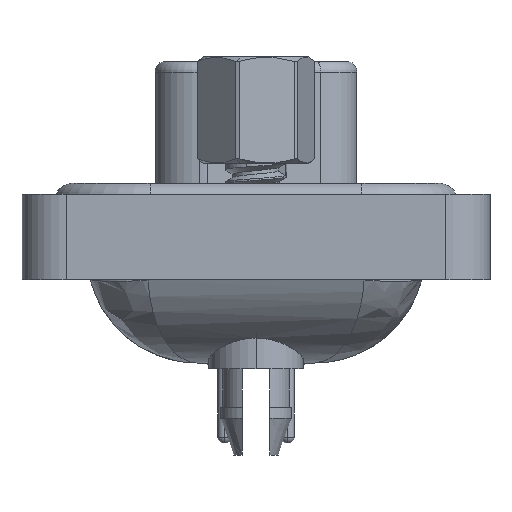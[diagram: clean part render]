
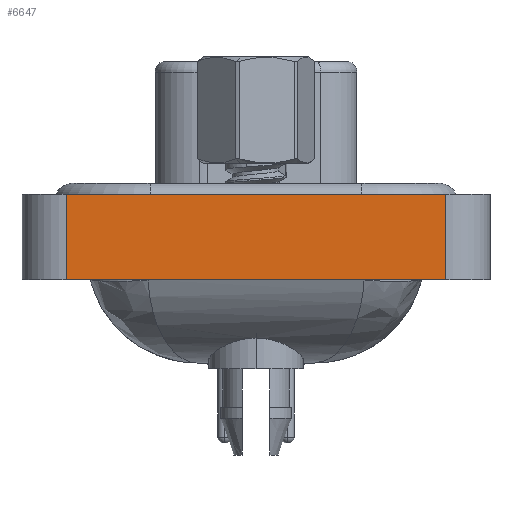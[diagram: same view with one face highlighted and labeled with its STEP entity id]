
A CAD part, left-side view. The second image highlights one B-rep face of the part: STEP entity #6647.
In plain terms, the highlighted planar face has unit normal (-1, 0, 0).
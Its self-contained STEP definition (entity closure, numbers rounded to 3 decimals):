
#2953 = EDGE_LOOP ( 'NONE', ( #7243, #8491, #27881, #7110 ) ) ;
#3103 = VERTEX_POINT ( 'NONE', #6133 ) ;
#4012 = FACE_OUTER_BOUND ( 'NONE', #2953, .T. ) ;
#4313 = CARTESIAN_POINT ( 'NONE',  ( -7.225, -8.55, -3.35 ) ) ;
#5384 = VECTOR ( 'NONE', #24375, 1000. ) ;
#6133 = CARTESIAN_POINT ( 'NONE',  ( -7.225, 8.55, -3.35 ) ) ;
#6647 = ADVANCED_FACE ( 'NONE', ( #4012 ), #12559, .T. ) ;
#6920 = EDGE_CURVE ( 'NONE', #3103, #19046, #24095, .T. ) ;
#7110 = ORIENTED_EDGE ( 'NONE', *, *, #6920, .T. ) ;
#7243 = ORIENTED_EDGE ( 'NONE', *, *, #10063, .T. ) ;
#7672 = VECTOR ( 'NONE', #8652, 1000. ) ;
#8030 = VERTEX_POINT ( 'NONE', #23807 ) ;
#8491 = ORIENTED_EDGE ( 'NONE', *, *, #16950, .F. ) ;
#8652 = DIRECTION ( 'NONE',  ( 0., 0., 1. ) ) ;
#8949 = LINE ( 'NONE', #17741, #7672 ) ;
#10063 = EDGE_CURVE ( 'NONE', #19046, #8030, #12764, .T. ) ;
#10428 = DIRECTION ( 'NONE',  ( 0., -1., 0. ) ) ;
#12515 = VERTEX_POINT ( 'NONE', #19476 ) ;
#12559 = PLANE ( 'NONE',  #23102 ) ;
#12764 = LINE ( 'NONE', #15368, #18325 ) ;
#12779 = CARTESIAN_POINT ( 'NONE',  ( -7.225, -8.55, -3.35 ) ) ;
#15249 = VECTOR ( 'NONE', #10428, 1000. ) ;
#15368 = CARTESIAN_POINT ( 'NONE',  ( -7.225, -8.55, -3.35 ) ) ;
#16910 = LINE ( 'NONE', #21262, #15249 ) ;
#16950 = EDGE_CURVE ( 'NONE', #12515, #8030, #16910, .T. ) ;
#17741 = CARTESIAN_POINT ( 'NONE',  ( -7.225, 8.55, -3.35 ) ) ;
#18325 = VECTOR ( 'NONE', #23892, 1000. ) ;
#19044 = CARTESIAN_POINT ( 'NONE',  ( -7.225, -8.55, -3.35 ) ) ;
#19046 = VERTEX_POINT ( 'NONE', #12779 ) ;
#19476 = CARTESIAN_POINT ( 'NONE',  ( -7.225, 8.55, 0.5 ) ) ;
#21210 = DIRECTION ( 'NONE',  ( -1., 0., 0. ) ) ;
#21262 = CARTESIAN_POINT ( 'NONE',  ( -7.225, -8.55, 0.5 ) ) ;
#21350 = DIRECTION ( 'NONE',  ( 0., 0., 1. ) ) ;
#22880 = EDGE_CURVE ( 'NONE', #3103, #12515, #8949, .T. ) ;
#23102 = AXIS2_PLACEMENT_3D ( 'NONE', #19044, #21210, #21350 ) ;
#23807 = CARTESIAN_POINT ( 'NONE',  ( -7.225, -8.55, 0.5 ) ) ;
#23892 = DIRECTION ( 'NONE',  ( 0., 0., 1. ) ) ;
#24095 = LINE ( 'NONE', #4313, #5384 ) ;
#24375 = DIRECTION ( 'NONE',  ( 0., -1., 0. ) ) ;
#27881 = ORIENTED_EDGE ( 'NONE', *, *, #22880, .F. ) ;
